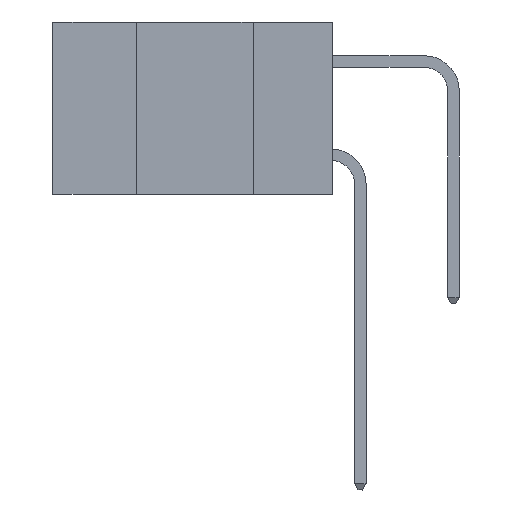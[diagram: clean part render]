
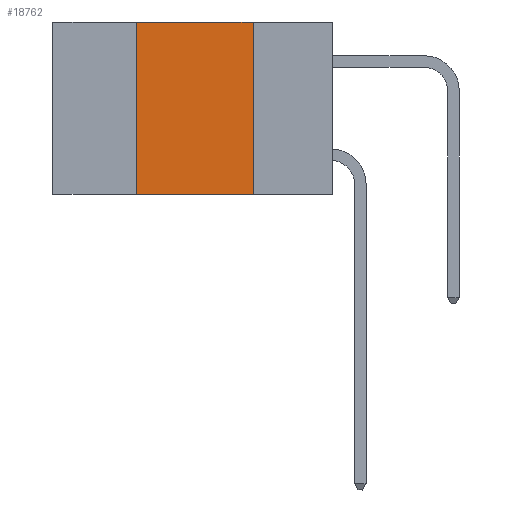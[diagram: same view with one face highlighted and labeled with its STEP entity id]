
A CAD part, left-side view. The second image highlights one B-rep face of the part: STEP entity #18762.
In plain terms, the highlighted planar face has unit normal (-1, 0, 0).
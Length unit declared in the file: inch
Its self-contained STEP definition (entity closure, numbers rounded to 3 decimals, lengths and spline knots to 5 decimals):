
#174 = ORIENTED_EDGE ( 'NONE', *, *, #6068, .F. ) ;
#203 = DIRECTION ( 'NONE',  ( 0., -1., 0. ) ) ;
#1033 = DIRECTION ( 'NONE',  ( 0., 0., -1. ) ) ;
#1057 = CARTESIAN_POINT ( 'NONE',  ( 0., 0.17, 0. ) ) ;
#2315 = VECTOR ( 'NONE', #11987, 39.37008 ) ;
#3019 = VERTEX_POINT ( 'NONE', #9114 ) ;
#5478 = DIRECTION ( 'NONE',  ( 1., 0., 0. ) ) ;
#5769 = CARTESIAN_POINT ( 'NONE',  ( 0., 0.17, 0. ) ) ;
#5970 = EDGE_CURVE ( 'NONE', #21955, #18726, #9226, .T. ) ;
#6068 = EDGE_CURVE ( 'NONE', #3019, #18237, #21148, .T. ) ;
#7175 = VECTOR ( 'NONE', #203, 39.37008 ) ;
#7211 = AXIS2_PLACEMENT_3D ( 'NONE', #14355, #5478, #17937 ) ;
#7398 = EDGE_LOOP ( 'NONE', ( #12100, #12679, #174, #14879 ) ) ;
#9114 = CARTESIAN_POINT ( 'NONE',  ( 0., 0.42, -0.37 ) ) ;
#9226 = LINE ( 'NONE', #1057, #18155 ) ;
#11987 = DIRECTION ( 'NONE',  ( 0., 0., 1. ) ) ;
#12100 = ORIENTED_EDGE ( 'NONE', *, *, #5970, .F. ) ;
#12123 = CARTESIAN_POINT ( 'NONE',  ( 0., 0.42, 0. ) ) ;
#12227 = DIRECTION ( 'NONE',  ( 0., -1., 0. ) ) ;
#12520 = LINE ( 'NONE', #12637, #7175 ) ;
#12531 = EDGE_CURVE ( 'NONE', #3019, #18726, #12520, .T. ) ;
#12637 = CARTESIAN_POINT ( 'NONE',  ( 0., 0.6, -0.37 ) ) ;
#12679 = ORIENTED_EDGE ( 'NONE', *, *, #19817, .F. ) ;
#13599 = LINE ( 'NONE', #14025, #19434 ) ;
#14025 = CARTESIAN_POINT ( 'NONE',  ( 0., 0.6, 0. ) ) ;
#14139 = CARTESIAN_POINT ( 'NONE',  ( 0., 0.17, -0.37 ) ) ;
#14355 = CARTESIAN_POINT ( 'NONE',  ( 0., 0.6, 0. ) ) ;
#14879 = ORIENTED_EDGE ( 'NONE', *, *, #12531, .T. ) ;
#16129 = PLANE ( 'NONE',  #7211 ) ;
#16957 = FACE_OUTER_BOUND ( 'NONE', #7398, .T. ) ;
#17937 = DIRECTION ( 'NONE',  ( 0., 0., -1. ) ) ;
#18155 = VECTOR ( 'NONE', #1033, 39.37008 ) ;
#18237 = VERTEX_POINT ( 'NONE', #18985 ) ;
#18726 = VERTEX_POINT ( 'NONE', #14139 ) ;
#18762 = ADVANCED_FACE ( 'NONE', ( #16957 ), #16129, .F. ) ;
#18985 = CARTESIAN_POINT ( 'NONE',  ( 0., 0.42, 0. ) ) ;
#19434 = VECTOR ( 'NONE', #12227, 39.37008 ) ;
#19817 = EDGE_CURVE ( 'NONE', #18237, #21955, #13599, .T. ) ;
#21148 = LINE ( 'NONE', #12123, #2315 ) ;
#21955 = VERTEX_POINT ( 'NONE', #5769 ) ;
